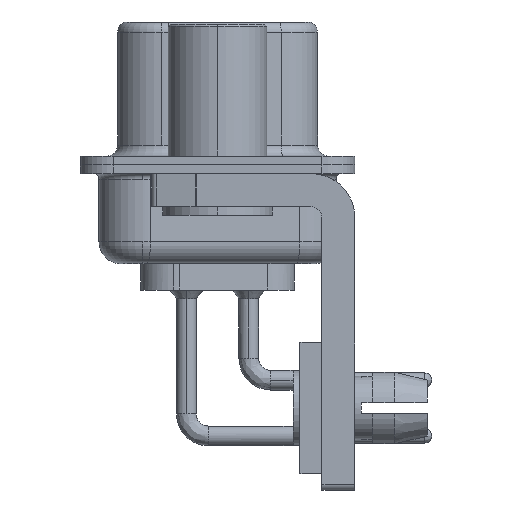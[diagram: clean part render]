
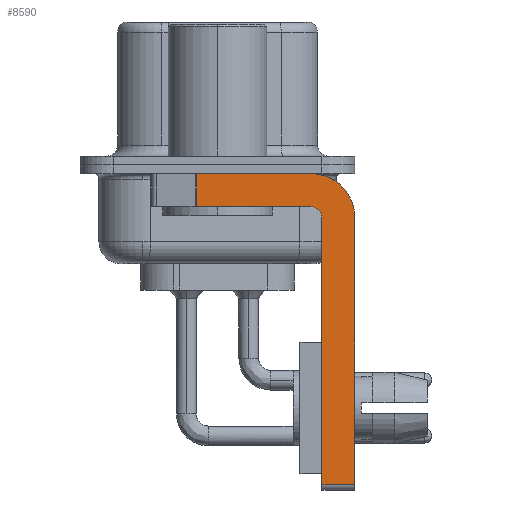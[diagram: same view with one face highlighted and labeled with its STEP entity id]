
A CAD part, left-side view. The second image highlights one B-rep face of the part: STEP entity #8590.
In plain terms, the highlighted planar face has unit normal (-1, 0, 0).
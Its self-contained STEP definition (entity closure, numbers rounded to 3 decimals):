
#43 = DIRECTION ( 'NONE',  ( 0., 0., -1. ) ) ;
#101 = CARTESIAN_POINT ( 'NONE',  ( -2.9, -6.25, -14.55 ) ) ;
#951 = AXIS2_PLACEMENT_3D ( 'NONE', #24121, #11757, #26230 ) ;
#1377 = CIRCLE ( 'NONE', #24725, 0.5 ) ;
#2022 = ORIENTED_EDGE ( 'NONE', *, *, #6624, .F. ) ;
#2564 = VECTOR ( 'NONE', #18830, 1000. ) ;
#2684 = PLANE ( 'NONE',  #13448 ) ;
#2820 = CARTESIAN_POINT ( 'NONE',  ( -2.9, -6.25, -2.4 ) ) ;
#2890 = CARTESIAN_POINT ( 'NONE',  ( -2.9, -4.25, -1.9 ) ) ;
#3306 = DIRECTION ( 'NONE',  ( 0., 0., 1. ) ) ;
#3331 = DIRECTION ( 'NONE',  ( 0., -1., 0. ) ) ;
#3360 = VERTEX_POINT ( 'NONE', #5114 ) ;
#3686 = VERTEX_POINT ( 'NONE', #7839 ) ;
#4111 = ORIENTED_EDGE ( 'NONE', *, *, #6530, .T. ) ;
#4198 = DIRECTION ( 'NONE',  ( -1., 0., 0. ) ) ;
#5114 = CARTESIAN_POINT ( 'NONE',  ( -2.9, -4.25, -0.4 ) ) ;
#5678 = EDGE_CURVE ( 'NONE', #3686, #8089, #14811, .T. ) ;
#6530 = EDGE_CURVE ( 'NONE', #14964, #24895, #20646, .T. ) ;
#6624 = EDGE_CURVE ( 'NONE', #9870, #24895, #12490, .T. ) ;
#7005 = DIRECTION ( 'NONE',  ( 0., 0., -1. ) ) ;
#7839 = CARTESIAN_POINT ( 'NONE',  ( -2.9, -4.25, -1.9 ) ) ;
#8089 = VERTEX_POINT ( 'NONE', #22036 ) ;
#8590 = ADVANCED_FACE ( 'NONE', ( #9894 ), #2684, .F. ) ;
#8642 = VECTOR ( 'NONE', #21750, 1000. ) ;
#8816 = EDGE_CURVE ( 'NONE', #15936, #3360, #15685, .T. ) ;
#8972 = CARTESIAN_POINT ( 'NONE',  ( -2.9, -4.75, -14.55 ) ) ;
#9253 = ORIENTED_EDGE ( 'NONE', *, *, #8816, .F. ) ;
#9870 = VERTEX_POINT ( 'NONE', #2820 ) ;
#9876 = EDGE_LOOP ( 'NONE', ( #9253, #22708, #23881, #14765, #17582, #4111, #2022, #12535 ) ) ;
#9894 = FACE_OUTER_BOUND ( 'NONE', #9876, .T. ) ;
#10432 = VECTOR ( 'NONE', #19237, 1000. ) ;
#11587 = CARTESIAN_POINT ( 'NONE',  ( -2.9, 0.978, -0.4 ) ) ;
#11757 = DIRECTION ( 'NONE',  ( 1., 0., 0. ) ) ;
#12083 = VERTEX_POINT ( 'NONE', #21401 ) ;
#12490 = LINE ( 'NONE', #14910, #18006 ) ;
#12535 = ORIENTED_EDGE ( 'NONE', *, *, #21363, .F. ) ;
#13448 = AXIS2_PLACEMENT_3D ( 'NONE', #17382, #19510, #7005 ) ;
#13833 = CARTESIAN_POINT ( 'NONE',  ( -2.9, 3., -0.4 ) ) ;
#13892 = EDGE_CURVE ( 'NONE', #14964, #12083, #16413, .T. ) ;
#14765 = ORIENTED_EDGE ( 'NONE', *, *, #16959, .F. ) ;
#14811 = LINE ( 'NONE', #2890, #8642 ) ;
#14910 = CARTESIAN_POINT ( 'NONE',  ( -2.9, -6.25, -2.4 ) ) ;
#14964 = VERTEX_POINT ( 'NONE', #8972 ) ;
#15031 = VECTOR ( 'NONE', #3331, 1000. ) ;
#15685 = LINE ( 'NONE', #13833, #15031 ) ;
#15936 = VERTEX_POINT ( 'NONE', #11587 ) ;
#16413 = LINE ( 'NONE', #20030, #21310 ) ;
#16717 = CARTESIAN_POINT ( 'NONE',  ( -2.9, -4.25, -14.55 ) ) ;
#16763 = CARTESIAN_POINT ( 'NONE',  ( -2.9, -4.25, -2.4 ) ) ;
#16959 = EDGE_CURVE ( 'NONE', #12083, #3686, #1377, .T. ) ;
#17382 = CARTESIAN_POINT ( 'NONE',  ( -2.9, -4.25, -2.4 ) ) ;
#17582 = ORIENTED_EDGE ( 'NONE', *, *, #13892, .F. ) ;
#18006 = VECTOR ( 'NONE', #43, 1000. ) ;
#18830 = DIRECTION ( 'NONE',  ( 0., -1., 0. ) ) ;
#18875 = DIRECTION ( 'NONE',  ( 0., 0., 1. ) ) ;
#19237 = DIRECTION ( 'NONE',  ( 0., 0., -1. ) ) ;
#19510 = DIRECTION ( 'NONE',  ( 1., 0., 0. ) ) ;
#20030 = CARTESIAN_POINT ( 'NONE',  ( -2.9, -4.75, -14.8 ) ) ;
#20646 = LINE ( 'NONE', #16717, #2564 ) ;
#21310 = VECTOR ( 'NONE', #3306, 1000. ) ;
#21363 = EDGE_CURVE ( 'NONE', #3360, #9870, #24784, .T. ) ;
#21401 = CARTESIAN_POINT ( 'NONE',  ( -2.9, -4.75, -2.4 ) ) ;
#21750 = DIRECTION ( 'NONE',  ( 0., 1., 0. ) ) ;
#22036 = CARTESIAN_POINT ( 'NONE',  ( -2.9, 0.978, -1.9 ) ) ;
#22708 = ORIENTED_EDGE ( 'NONE', *, *, #24937, .T. ) ;
#23350 = CARTESIAN_POINT ( 'NONE',  ( -2.9, 0.978, -1.9 ) ) ;
#23881 = ORIENTED_EDGE ( 'NONE', *, *, #5678, .F. ) ;
#24121 = CARTESIAN_POINT ( 'NONE',  ( -2.9, -4.25, -2.4 ) ) ;
#24725 = AXIS2_PLACEMENT_3D ( 'NONE', #16763, #4198, #18875 ) ;
#24784 = CIRCLE ( 'NONE', #951, 2. ) ;
#24895 = VERTEX_POINT ( 'NONE', #101 ) ;
#24937 = EDGE_CURVE ( 'NONE', #15936, #8089, #26941, .T. ) ;
#26230 = DIRECTION ( 'NONE',  ( 0., 0., -1. ) ) ;
#26941 = LINE ( 'NONE', #23350, #10432 ) ;
